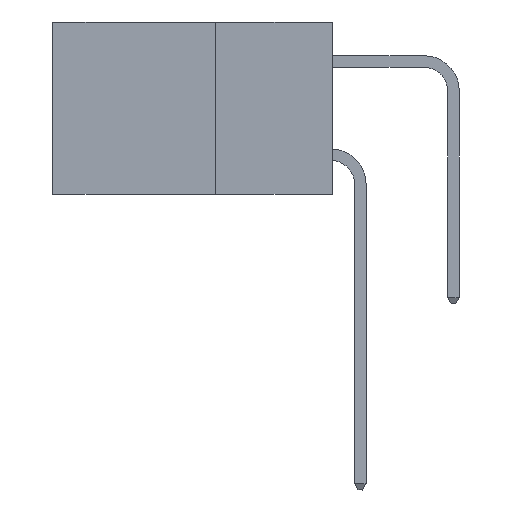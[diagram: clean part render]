
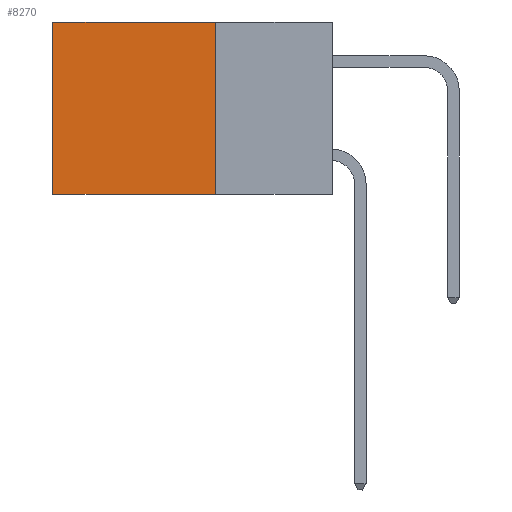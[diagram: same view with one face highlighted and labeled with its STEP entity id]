
A CAD part, left-side view. The second image highlights one B-rep face of the part: STEP entity #8270.
In plain terms, the highlighted planar face has unit normal (-1, 0, 0).
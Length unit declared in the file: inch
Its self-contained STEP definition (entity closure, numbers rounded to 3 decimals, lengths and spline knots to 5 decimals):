
#27 = CARTESIAN_POINT ( 'NONE',  ( 0.2615, 0.25, -0.37 ) ) ;
#31 = DIRECTION ( 'NONE',  ( 1., 0., 0. ) ) ;
#879 = LINE ( 'NONE', #3391, #8241 ) ;
#1059 = FACE_OUTER_BOUND ( 'NONE', #11385, .T. ) ;
#1457 = CARTESIAN_POINT ( 'NONE',  ( 0.2615, 0.25, -0.37 ) ) ;
#1489 = EDGE_CURVE ( 'NONE', #6540, #10127, #8246, .T. ) ;
#1901 = CARTESIAN_POINT ( 'NONE',  ( 0.2615, 0.25, -0.37 ) ) ;
#1949 = CARTESIAN_POINT ( 'NONE',  ( 0.2615, 0.6, 0. ) ) ;
#2149 = AXIS2_PLACEMENT_3D ( 'NONE', #1901, #31, #2850 ) ;
#2400 = VERTEX_POINT ( 'NONE', #1949 ) ;
#2526 = LINE ( 'NONE', #1457, #6717 ) ;
#2850 = DIRECTION ( 'NONE',  ( 0., 0., -1. ) ) ;
#2961 = CARTESIAN_POINT ( 'NONE',  ( 0.2615, 0.25, -0.37 ) ) ;
#3391 = CARTESIAN_POINT ( 'NONE',  ( 0.2615, 0.6, -0.37 ) ) ;
#3690 = DIRECTION ( 'NONE',  ( 0., 0., -1. ) ) ;
#3759 = ORIENTED_EDGE ( 'NONE', *, *, #9188, .T. ) ;
#4082 = DIRECTION ( 'NONE',  ( 0., 1., 0. ) ) ;
#4904 = CARTESIAN_POINT ( 'NONE',  ( 0.2615, 0.6, -0.37 ) ) ;
#5467 = VECTOR ( 'NONE', #3690, 39.37008 ) ;
#6017 = ORIENTED_EDGE ( 'NONE', *, *, #1489, .F. ) ;
#6540 = VERTEX_POINT ( 'NONE', #6588 ) ;
#6575 = PLANE ( 'NONE',  #2149 ) ;
#6588 = CARTESIAN_POINT ( 'NONE',  ( 0.2615, 0.25, 0. ) ) ;
#6645 = DIRECTION ( 'NONE',  ( 0., 1., 0. ) ) ;
#6717 = VECTOR ( 'NONE', #4082, 39.37008 ) ;
#6803 = EDGE_CURVE ( 'NONE', #2400, #7989, #879, .T. ) ;
#7156 = EDGE_CURVE ( 'NONE', #10127, #7989, #2526, .T. ) ;
#7989 = VERTEX_POINT ( 'NONE', #4904 ) ;
#8085 = ORIENTED_EDGE ( 'NONE', *, *, #7156, .F. ) ;
#8241 = VECTOR ( 'NONE', #11804, 39.37008 ) ;
#8246 = LINE ( 'NONE', #27, #5467 ) ;
#8270 = ADVANCED_FACE ( 'NONE', ( #1059 ), #6575, .F. ) ;
#9188 = EDGE_CURVE ( 'NONE', #6540, #2400, #11075, .T. ) ;
#10127 = VERTEX_POINT ( 'NONE', #2961 ) ;
#10193 = CARTESIAN_POINT ( 'NONE',  ( 0.2615, 0.25, 0. ) ) ;
#10367 = VECTOR ( 'NONE', #6645, 39.37008 ) ;
#11075 = LINE ( 'NONE', #10193, #10367 ) ;
#11385 = EDGE_LOOP ( 'NONE', ( #11696, #8085, #6017, #3759 ) ) ;
#11696 = ORIENTED_EDGE ( 'NONE', *, *, #6803, .T. ) ;
#11804 = DIRECTION ( 'NONE',  ( 0., 0., -1. ) ) ;
